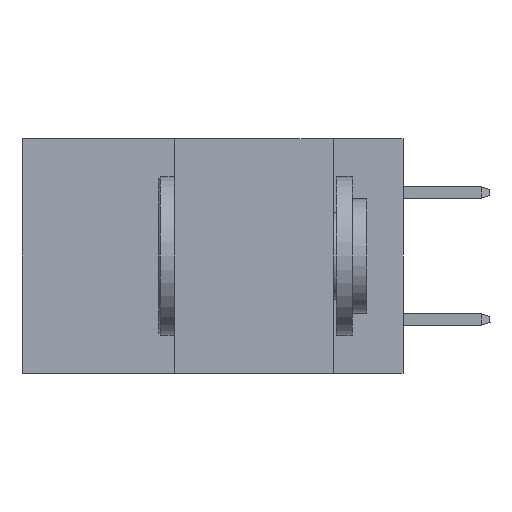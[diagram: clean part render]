
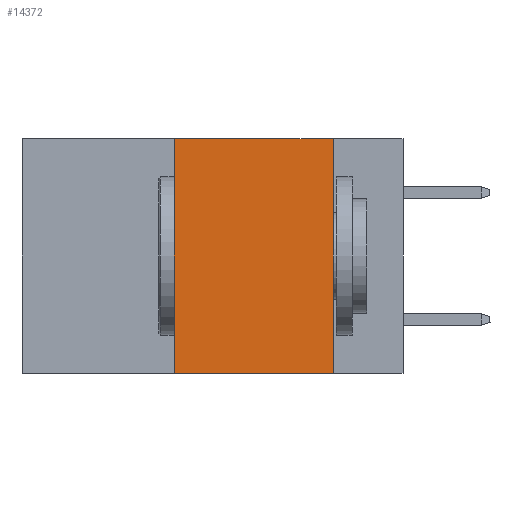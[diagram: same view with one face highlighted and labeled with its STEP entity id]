
A CAD part, left-side view. The second image highlights one B-rep face of the part: STEP entity #14372.
In plain terms, the highlighted planar face has unit normal (-1, 0, 0).
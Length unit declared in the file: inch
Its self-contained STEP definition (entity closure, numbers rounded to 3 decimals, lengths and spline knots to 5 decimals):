
#33 = ORIENTED_EDGE ( 'NONE', *, *, #17269, .F. ) ;
#162 = CARTESIAN_POINT ( 'NONE',  ( 0., 0.36, -0.37 ) ) ;
#298 = VECTOR ( 'NONE', #6066, 39.37008 ) ;
#400 = PLANE ( 'NONE',  #6684 ) ;
#487 = DIRECTION ( 'NONE',  ( 1., 0., 0. ) ) ;
#496 = CARTESIAN_POINT ( 'NONE',  ( 0., 0.6, 0. ) ) ;
#535 = DIRECTION ( 'NONE',  ( 0., 0., -1. ) ) ;
#551 = ORIENTED_EDGE ( 'NONE', *, *, #17375, .F. ) ;
#5140 = CARTESIAN_POINT ( 'NONE',  ( 0., 0.11, 0. ) ) ;
#5448 = VERTEX_POINT ( 'NONE', #6033 ) ;
#6033 = CARTESIAN_POINT ( 'NONE',  ( 0., 0.11, 0. ) ) ;
#6066 = DIRECTION ( 'NONE',  ( 0., -1., 0. ) ) ;
#6394 = LINE ( 'NONE', #5140, #6674 ) ;
#6674 = VECTOR ( 'NONE', #535, 39.37008 ) ;
#6684 = AXIS2_PLACEMENT_3D ( 'NONE', #9299, #487, #7882 ) ;
#6756 = VECTOR ( 'NONE', #10398, 39.37008 ) ;
#7462 = VERTEX_POINT ( 'NONE', #16346 ) ;
#7512 = LINE ( 'NONE', #14666, #6756 ) ;
#7781 = FACE_OUTER_BOUND ( 'NONE', #11270, .T. ) ;
#7882 = DIRECTION ( 'NONE',  ( 0., 0., -1. ) ) ;
#8945 = VERTEX_POINT ( 'NONE', #17466 ) ;
#9299 = CARTESIAN_POINT ( 'NONE',  ( 0., 0.6, 0. ) ) ;
#9516 = VECTOR ( 'NONE', #10572, 39.37008 ) ;
#10398 = DIRECTION ( 'NONE',  ( 0., 0., 1. ) ) ;
#10572 = DIRECTION ( 'NONE',  ( 0., -1., 0. ) ) ;
#11270 = EDGE_LOOP ( 'NONE', ( #17708, #551, #33, #17299 ) ) ;
#11974 = LINE ( 'NONE', #16446, #298 ) ;
#12438 = EDGE_CURVE ( 'NONE', #5448, #8945, #6394, .T. ) ;
#12697 = VERTEX_POINT ( 'NONE', #162 ) ;
#13510 = LINE ( 'NONE', #496, #9516 ) ;
#14372 = ADVANCED_FACE ( 'NONE', ( #7781 ), #400, .F. ) ;
#14666 = CARTESIAN_POINT ( 'NONE',  ( 0., 0.36, 0. ) ) ;
#15761 = EDGE_CURVE ( 'NONE', #12697, #8945, #11974, .T. ) ;
#16346 = CARTESIAN_POINT ( 'NONE',  ( 0., 0.36, 0. ) ) ;
#16446 = CARTESIAN_POINT ( 'NONE',  ( 0., 0.6, -0.37 ) ) ;
#17269 = EDGE_CURVE ( 'NONE', #12697, #7462, #7512, .T. ) ;
#17299 = ORIENTED_EDGE ( 'NONE', *, *, #15761, .T. ) ;
#17375 = EDGE_CURVE ( 'NONE', #7462, #5448, #13510, .T. ) ;
#17466 = CARTESIAN_POINT ( 'NONE',  ( 0., 0.11, -0.37 ) ) ;
#17708 = ORIENTED_EDGE ( 'NONE', *, *, #12438, .F. ) ;
